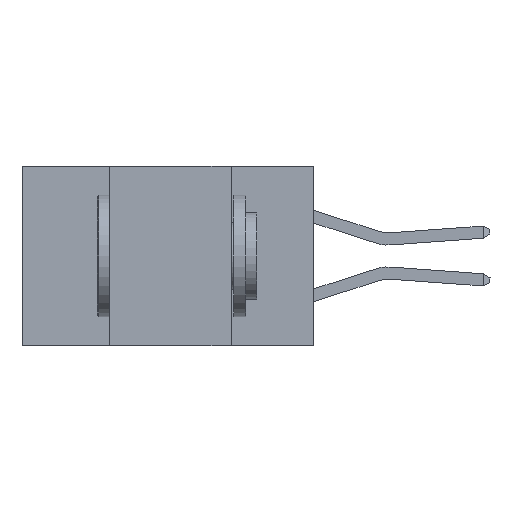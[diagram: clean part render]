
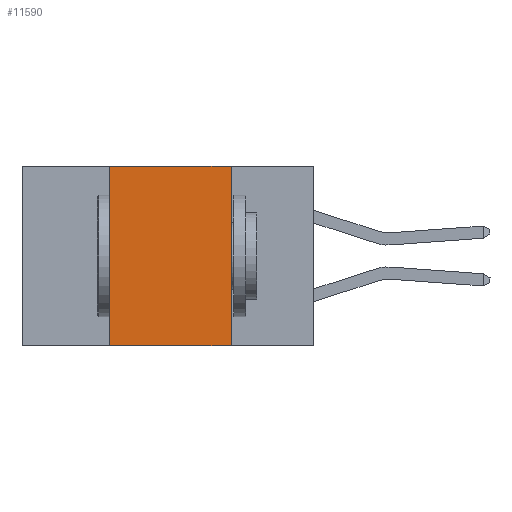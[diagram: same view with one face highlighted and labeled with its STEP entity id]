
A CAD part, left-side view. The second image highlights one B-rep face of the part: STEP entity #11590.
In plain terms, the highlighted planar face has unit normal (-1, 0, 0).
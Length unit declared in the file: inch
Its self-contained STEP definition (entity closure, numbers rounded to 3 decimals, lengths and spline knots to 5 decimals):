
#119 = DIRECTION ( 'NONE',  ( 0., 0., -1. ) ) ;
#156 = CARTESIAN_POINT ( 'NONE',  ( 0., 0.17, 0. ) ) ;
#529 = VECTOR ( 'NONE', #2078, 39.37008 ) ;
#594 = DIRECTION ( 'NONE',  ( 0., 0., -1. ) ) ;
#664 = FACE_OUTER_BOUND ( 'NONE', #4220, .T. ) ;
#668 = VERTEX_POINT ( 'NONE', #5692 ) ;
#932 = ORIENTED_EDGE ( 'NONE', *, *, #7775, .F. ) ;
#1149 = CARTESIAN_POINT ( 'NONE',  ( 0., 0.42, 0. ) ) ;
#1352 = EDGE_CURVE ( 'NONE', #6437, #2793, #6687, .T. ) ;
#2054 = VERTEX_POINT ( 'NONE', #3675 ) ;
#2078 = DIRECTION ( 'NONE',  ( 0., 0., 1. ) ) ;
#2259 = CARTESIAN_POINT ( 'NONE',  ( 0., 0.6, 0. ) ) ;
#2361 = EDGE_CURVE ( 'NONE', #2054, #2793, #10606, .T. ) ;
#2793 = VERTEX_POINT ( 'NONE', #9825 ) ;
#2963 = LINE ( 'NONE', #1149, #529 ) ;
#3649 = VECTOR ( 'NONE', #119, 39.37008 ) ;
#3675 = CARTESIAN_POINT ( 'NONE',  ( 0., 0.17, 0. ) ) ;
#3732 = VECTOR ( 'NONE', #7533, 39.37008 ) ;
#4220 = EDGE_LOOP ( 'NONE', ( #8079, #5228, #932, #10903 ) ) ;
#4263 = VECTOR ( 'NONE', #9768, 39.37008 ) ;
#5228 = ORIENTED_EDGE ( 'NONE', *, *, #6004, .F. ) ;
#5692 = CARTESIAN_POINT ( 'NONE',  ( 0., 0.42, 0. ) ) ;
#6004 = EDGE_CURVE ( 'NONE', #668, #2054, #10947, .T. ) ;
#6023 = CARTESIAN_POINT ( 'NONE',  ( 0., 0.42, -0.37 ) ) ;
#6050 = DIRECTION ( 'NONE',  ( 1., 0., 0. ) ) ;
#6437 = VERTEX_POINT ( 'NONE', #6023 ) ;
#6687 = LINE ( 'NONE', #9814, #4263 ) ;
#7324 = AXIS2_PLACEMENT_3D ( 'NONE', #11466, #6050, #594 ) ;
#7533 = DIRECTION ( 'NONE',  ( 0., -1., 0. ) ) ;
#7775 = EDGE_CURVE ( 'NONE', #6437, #668, #2963, .T. ) ;
#8079 = ORIENTED_EDGE ( 'NONE', *, *, #2361, .F. ) ;
#9768 = DIRECTION ( 'NONE',  ( 0., -1., 0. ) ) ;
#9814 = CARTESIAN_POINT ( 'NONE',  ( 0., 0.6, -0.37 ) ) ;
#9825 = CARTESIAN_POINT ( 'NONE',  ( 0., 0.17, -0.37 ) ) ;
#10589 = PLANE ( 'NONE',  #7324 ) ;
#10606 = LINE ( 'NONE', #156, #3649 ) ;
#10903 = ORIENTED_EDGE ( 'NONE', *, *, #1352, .T. ) ;
#10947 = LINE ( 'NONE', #2259, #3732 ) ;
#11466 = CARTESIAN_POINT ( 'NONE',  ( 0., 0.6, 0. ) ) ;
#11590 = ADVANCED_FACE ( 'NONE', ( #664 ), #10589, .F. ) ;
